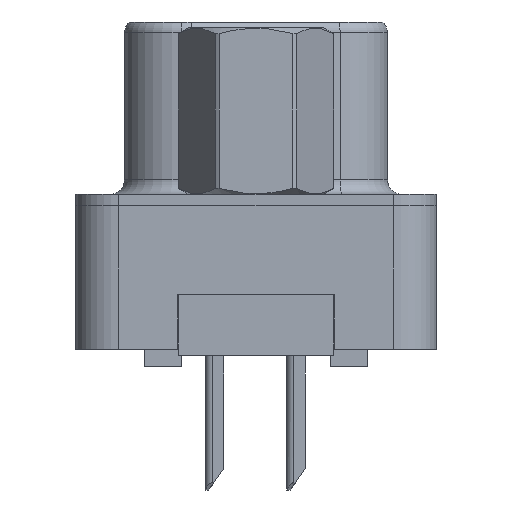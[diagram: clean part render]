
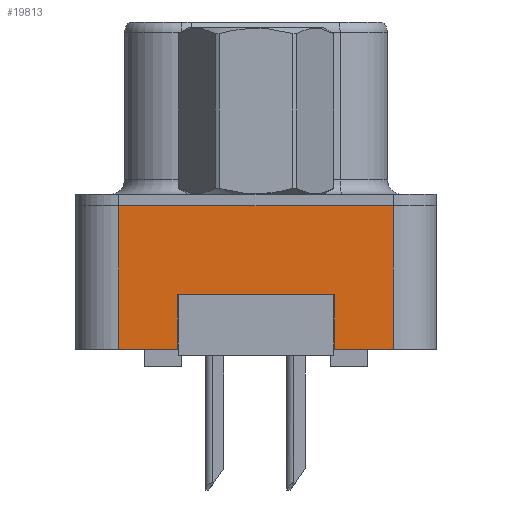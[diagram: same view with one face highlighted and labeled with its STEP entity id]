
A CAD part, left-side view. The second image highlights one B-rep face of the part: STEP entity #19813.
In plain terms, the highlighted planar face has unit normal (-1, 0, 0).
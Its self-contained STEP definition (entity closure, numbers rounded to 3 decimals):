
#57 = EDGE_CURVE ( 'NONE', #11918, #10654, #3614, .T. ) ;
#127 = ORIENTED_EDGE ( 'NONE', *, *, #15205, .T. ) ;
#466 = VECTOR ( 'NONE', #3828, 1000. ) ;
#934 = CARTESIAN_POINT ( 'NONE',  ( -2.91, -4.775, -5. ) ) ;
#1008 = CARTESIAN_POINT ( 'NONE',  ( -2.91, -4.775, 0. ) ) ;
#1236 = CARTESIAN_POINT ( 'NONE',  ( -2.91, -2.75, -5. ) ) ;
#1420 = DIRECTION ( 'NONE',  ( 0., 0., -1. ) ) ;
#2096 = CARTESIAN_POINT ( 'NONE',  ( -2.91, 2.75, -3.1 ) ) ;
#2790 = CARTESIAN_POINT ( 'NONE',  ( -2.91, 2.75, -3.1 ) ) ;
#2839 = CARTESIAN_POINT ( 'NONE',  ( -2.91, -4.775, -5. ) ) ;
#3409 = VECTOR ( 'NONE', #12134, 1000. ) ;
#3614 = LINE ( 'NONE', #2096, #466 ) ;
#3828 = DIRECTION ( 'NONE',  ( 0., 0., -1. ) ) ;
#3905 = DIRECTION ( 'NONE',  ( 0., 1., 0. ) ) ;
#4051 = EDGE_CURVE ( 'NONE', #15019, #10654, #18372, .T. ) ;
#4583 = EDGE_CURVE ( 'NONE', #9731, #11918, #10432, .T. ) ;
#4589 = CARTESIAN_POINT ( 'NONE',  ( -2.91, -4.775, -5. ) ) ;
#4831 = EDGE_LOOP ( 'NONE', ( #13087, #127, #7068, #16770, #14963, #14044, #4873, #4984 ) ) ;
#4873 = ORIENTED_EDGE ( 'NONE', *, *, #57, .F. ) ;
#4925 = LINE ( 'NONE', #18814, #19222 ) ;
#4958 = CARTESIAN_POINT ( 'NONE',  ( -2.91, 2.75, -3.1 ) ) ;
#4984 = ORIENTED_EDGE ( 'NONE', *, *, #4583, .F. ) ;
#5066 = CARTESIAN_POINT ( 'NONE',  ( -2.91, 4.775, -5. ) ) ;
#5363 = DIRECTION ( 'NONE',  ( 0., -1., 0. ) ) ;
#5582 = VERTEX_POINT ( 'NONE', #1008 ) ;
#6004 = CARTESIAN_POINT ( 'NONE',  ( -2.91, -4.775, 0. ) ) ;
#6059 = DIRECTION ( 'NONE',  ( -1., 0., 0. ) ) ;
#6867 = VECTOR ( 'NONE', #10710, 1000. ) ;
#7013 = EDGE_CURVE ( 'NONE', #7148, #5582, #13751, .T. ) ;
#7068 = ORIENTED_EDGE ( 'NONE', *, *, #15862, .T. ) ;
#7148 = VERTEX_POINT ( 'NONE', #7481 ) ;
#7481 = CARTESIAN_POINT ( 'NONE',  ( -2.91, 4.775, 0. ) ) ;
#7952 = DIRECTION ( 'NONE',  ( 0., 0., 1. ) ) ;
#8091 = EDGE_CURVE ( 'NONE', #15019, #7148, #17147, .T. ) ;
#8317 = AXIS2_PLACEMENT_3D ( 'NONE', #18525, #6059, #7952 ) ;
#9731 = VERTEX_POINT ( 'NONE', #11542 ) ;
#10432 = LINE ( 'NONE', #2790, #14266 ) ;
#10654 = VERTEX_POINT ( 'NONE', #14686 ) ;
#10710 = DIRECTION ( 'NONE',  ( 0., -1., 0. ) ) ;
#10880 = FACE_OUTER_BOUND ( 'NONE', #4831, .T. ) ;
#11393 = CARTESIAN_POINT ( 'NONE',  ( -2.91, 4.775, -5. ) ) ;
#11542 = CARTESIAN_POINT ( 'NONE',  ( -2.91, -2.75, -3.1 ) ) ;
#11918 = VERTEX_POINT ( 'NONE', #4958 ) ;
#12134 = DIRECTION ( 'NONE',  ( 0., -1., 0. ) ) ;
#12293 = CARTESIAN_POINT ( 'NONE',  ( -2.91, -2.75, -3.1 ) ) ;
#12328 = VERTEX_POINT ( 'NONE', #2839 ) ;
#12381 = VECTOR ( 'NONE', #19146, 1000. ) ;
#13087 = ORIENTED_EDGE ( 'NONE', *, *, #14028, .T. ) ;
#13751 = LINE ( 'NONE', #6004, #3409 ) ;
#13806 = PLANE ( 'NONE',  #8317 ) ;
#14014 = VERTEX_POINT ( 'NONE', #1236 ) ;
#14028 = EDGE_CURVE ( 'NONE', #9731, #14014, #19736, .T. ) ;
#14044 = ORIENTED_EDGE ( 'NONE', *, *, #4051, .T. ) ;
#14056 = VECTOR ( 'NONE', #5363, 1000. ) ;
#14266 = VECTOR ( 'NONE', #3905, 1000. ) ;
#14273 = DIRECTION ( 'NONE',  ( 0., 0., 1. ) ) ;
#14686 = CARTESIAN_POINT ( 'NONE',  ( -2.91, 2.75, -5. ) ) ;
#14963 = ORIENTED_EDGE ( 'NONE', *, *, #8091, .F. ) ;
#15019 = VERTEX_POINT ( 'NONE', #11393 ) ;
#15205 = EDGE_CURVE ( 'NONE', #14014, #12328, #19159, .T. ) ;
#15637 = VECTOR ( 'NONE', #1420, 1000. ) ;
#15862 = EDGE_CURVE ( 'NONE', #12328, #5582, #4925, .T. ) ;
#16770 = ORIENTED_EDGE ( 'NONE', *, *, #7013, .F. ) ;
#17147 = LINE ( 'NONE', #5066, #12381 ) ;
#18372 = LINE ( 'NONE', #4589, #6867 ) ;
#18525 = CARTESIAN_POINT ( 'NONE',  ( -2.91, -4.775, -5. ) ) ;
#18814 = CARTESIAN_POINT ( 'NONE',  ( -2.91, -4.775, -5. ) ) ;
#19146 = DIRECTION ( 'NONE',  ( 0., 0., 1. ) ) ;
#19159 = LINE ( 'NONE', #934, #14056 ) ;
#19222 = VECTOR ( 'NONE', #14273, 1000. ) ;
#19736 = LINE ( 'NONE', #12293, #15637 ) ;
#19813 = ADVANCED_FACE ( 'NONE', ( #10880 ), #13806, .T. ) ;
